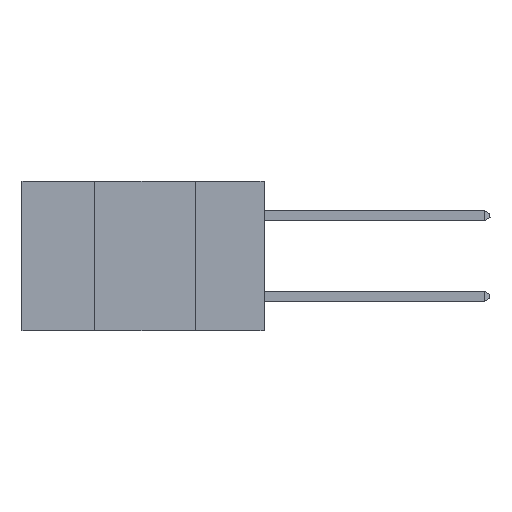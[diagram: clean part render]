
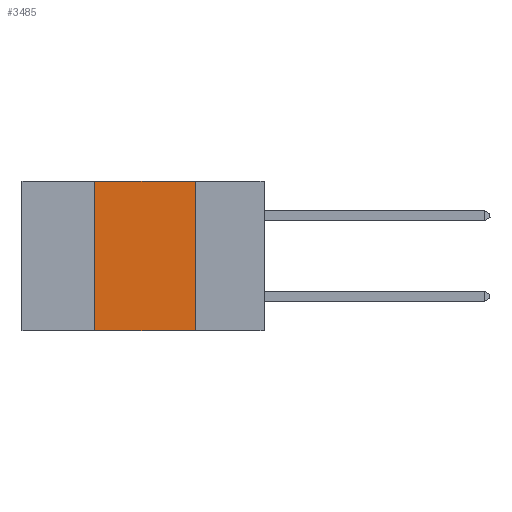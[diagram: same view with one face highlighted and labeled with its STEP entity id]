
A CAD part, left-side view. The second image highlights one B-rep face of the part: STEP entity #3485.
In plain terms, the highlighted planar face has unit normal (-1, 0, 0).
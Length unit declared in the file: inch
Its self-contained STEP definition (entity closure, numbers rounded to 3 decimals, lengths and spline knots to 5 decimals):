
#497 = LINE ( 'NONE', #10282, #9541 ) ;
#510 = DIRECTION ( 'NONE',  ( 0., 0., -1. ) ) ;
#558 = CARTESIAN_POINT ( 'NONE',  ( 0., 0.6, 0. ) ) ;
#684 = EDGE_CURVE ( 'NONE', #1280, #10004, #2019, .T. ) ;
#1117 = FACE_OUTER_BOUND ( 'NONE', #10716, .T. ) ;
#1156 = CARTESIAN_POINT ( 'NONE',  ( 0., 0.6, -0.37 ) ) ;
#1197 = DIRECTION ( 'NONE',  ( 0., 0., 1. ) ) ;
#1280 = VERTEX_POINT ( 'NONE', #8713 ) ;
#1870 = VERTEX_POINT ( 'NONE', #10015 ) ;
#1961 = AXIS2_PLACEMENT_3D ( 'NONE', #558, #2591, #510 ) ;
#2019 = LINE ( 'NONE', #1156, #6991 ) ;
#2591 = DIRECTION ( 'NONE',  ( 1., 0., 0. ) ) ;
#3130 = DIRECTION ( 'NONE',  ( 0., 0., -1. ) ) ;
#3485 = ADVANCED_FACE ( 'NONE', ( #1117 ), #9719, .F. ) ;
#3746 = EDGE_CURVE ( 'NONE', #5708, #1870, #7544, .T. ) ;
#5708 = VERTEX_POINT ( 'NONE', #8474 ) ;
#5749 = VECTOR ( 'NONE', #1197, 39.37008 ) ;
#6760 = DIRECTION ( 'NONE',  ( 0., -1., 0. ) ) ;
#6911 = ORIENTED_EDGE ( 'NONE', *, *, #12229, .F. ) ;
#6991 = VECTOR ( 'NONE', #12610, 39.37008 ) ;
#7467 = ORIENTED_EDGE ( 'NONE', *, *, #684, .T. ) ;
#7544 = LINE ( 'NONE', #8731, #9982 ) ;
#8474 = CARTESIAN_POINT ( 'NONE',  ( 0., 0.42, 0. ) ) ;
#8713 = CARTESIAN_POINT ( 'NONE',  ( 0., 0.42, -0.37 ) ) ;
#8731 = CARTESIAN_POINT ( 'NONE',  ( 0., 0.6, 0. ) ) ;
#8793 = EDGE_CURVE ( 'NONE', #1870, #10004, #497, .T. ) ;
#9541 = VECTOR ( 'NONE', #3130, 39.37008 ) ;
#9663 = CARTESIAN_POINT ( 'NONE',  ( 0., 0.17, -0.37 ) ) ;
#9719 = PLANE ( 'NONE',  #1961 ) ;
#9982 = VECTOR ( 'NONE', #6760, 39.37008 ) ;
#10004 = VERTEX_POINT ( 'NONE', #9663 ) ;
#10015 = CARTESIAN_POINT ( 'NONE',  ( 0., 0.17, 0. ) ) ;
#10282 = CARTESIAN_POINT ( 'NONE',  ( 0., 0.17, 0. ) ) ;
#10716 = EDGE_LOOP ( 'NONE', ( #11879, #11147, #6911, #7467 ) ) ;
#11147 = ORIENTED_EDGE ( 'NONE', *, *, #3746, .F. ) ;
#11488 = CARTESIAN_POINT ( 'NONE',  ( 0., 0.42, 0. ) ) ;
#11879 = ORIENTED_EDGE ( 'NONE', *, *, #8793, .F. ) ;
#11990 = LINE ( 'NONE', #11488, #5749 ) ;
#12229 = EDGE_CURVE ( 'NONE', #1280, #5708, #11990, .T. ) ;
#12610 = DIRECTION ( 'NONE',  ( 0., -1., 0. ) ) ;
